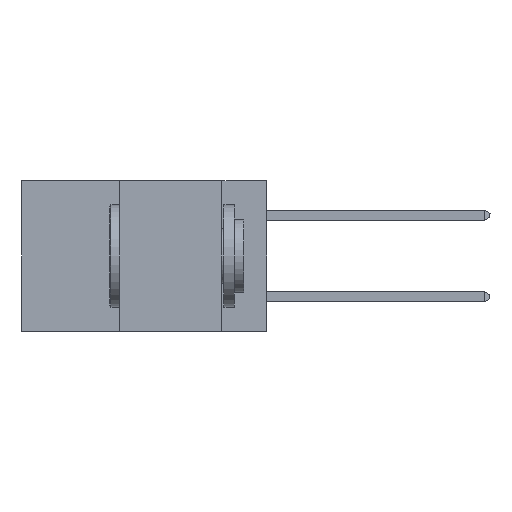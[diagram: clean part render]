
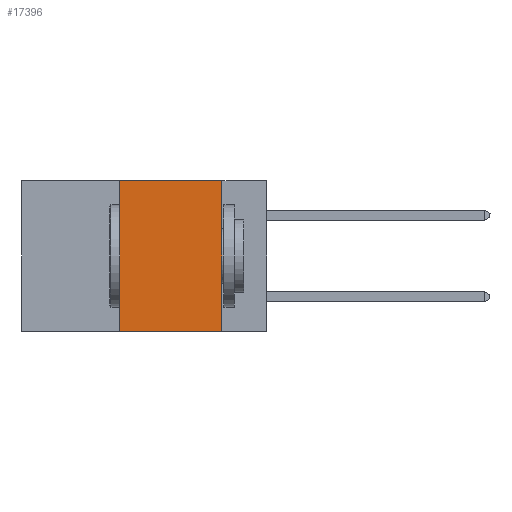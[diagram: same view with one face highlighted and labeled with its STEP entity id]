
A CAD part, left-side view. The second image highlights one B-rep face of the part: STEP entity #17396.
In plain terms, the highlighted planar face has unit normal (-1, 0, 0).
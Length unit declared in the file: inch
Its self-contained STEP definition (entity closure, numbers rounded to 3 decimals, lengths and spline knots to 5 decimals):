
#2334 = CARTESIAN_POINT ( 'NONE',  ( 0., 0.36, 0. ) ) ;
#4861 = CARTESIAN_POINT ( 'NONE',  ( 0., 0.11, 0. ) ) ;
#4969 = EDGE_CURVE ( 'NONE', #29195, #35740, #26469, .T. ) ;
#6721 = ORIENTED_EDGE ( 'NONE', *, *, #21225, .T. ) ;
#7838 = AXIS2_PLACEMENT_3D ( 'NONE', #13128, #24229, #13382 ) ;
#7898 = VECTOR ( 'NONE', #19766, 39.37008 ) ;
#9435 = CARTESIAN_POINT ( 'NONE',  ( 0., 0.6, -0.37 ) ) ;
#9792 = VECTOR ( 'NONE', #34978, 39.37008 ) ;
#11509 = EDGE_CURVE ( 'NONE', #18453, #33616, #29456, .T. ) ;
#12210 = ORIENTED_EDGE ( 'NONE', *, *, #21300, .F. ) ;
#13128 = CARTESIAN_POINT ( 'NONE',  ( 0., 0.6, 0. ) ) ;
#13363 = VECTOR ( 'NONE', #32520, 39.37008 ) ;
#13382 = DIRECTION ( 'NONE',  ( 0., 0., -1. ) ) ;
#15125 = LINE ( 'NONE', #26725, #9792 ) ;
#16374 = EDGE_LOOP ( 'NONE', ( #17284, #12210, #18006, #6721 ) ) ;
#17284 = ORIENTED_EDGE ( 'NONE', *, *, #11509, .F. ) ;
#17396 = ADVANCED_FACE ( 'NONE', ( #17589 ), #27075, .F. ) ;
#17589 = FACE_OUTER_BOUND ( 'NONE', #16374, .T. ) ;
#17900 = CARTESIAN_POINT ( 'NONE',  ( 0., 0.36, 0. ) ) ;
#18006 = ORIENTED_EDGE ( 'NONE', *, *, #4969, .F. ) ;
#18453 = VERTEX_POINT ( 'NONE', #4861 ) ;
#19766 = DIRECTION ( 'NONE',  ( 0., 0., 1. ) ) ;
#21225 = EDGE_CURVE ( 'NONE', #29195, #33616, #34067, .T. ) ;
#21300 = EDGE_CURVE ( 'NONE', #35740, #18453, #15125, .T. ) ;
#22863 = VECTOR ( 'NONE', #25035, 39.37008 ) ;
#24229 = DIRECTION ( 'NONE',  ( 1., 0., 0. ) ) ;
#25035 = DIRECTION ( 'NONE',  ( 0., 0., -1. ) ) ;
#26469 = LINE ( 'NONE', #2334, #7898 ) ;
#26725 = CARTESIAN_POINT ( 'NONE',  ( 0., 0.6, 0. ) ) ;
#27075 = PLANE ( 'NONE',  #7838 ) ;
#29195 = VERTEX_POINT ( 'NONE', #35035 ) ;
#29456 = LINE ( 'NONE', #36320, #22863 ) ;
#32520 = DIRECTION ( 'NONE',  ( 0., -1., 0. ) ) ;
#32695 = CARTESIAN_POINT ( 'NONE',  ( 0., 0.11, -0.37 ) ) ;
#33616 = VERTEX_POINT ( 'NONE', #32695 ) ;
#34067 = LINE ( 'NONE', #9435, #13363 ) ;
#34978 = DIRECTION ( 'NONE',  ( 0., -1., 0. ) ) ;
#35035 = CARTESIAN_POINT ( 'NONE',  ( 0., 0.36, -0.37 ) ) ;
#35740 = VERTEX_POINT ( 'NONE', #17900 ) ;
#36320 = CARTESIAN_POINT ( 'NONE',  ( 0., 0.11, 0. ) ) ;
